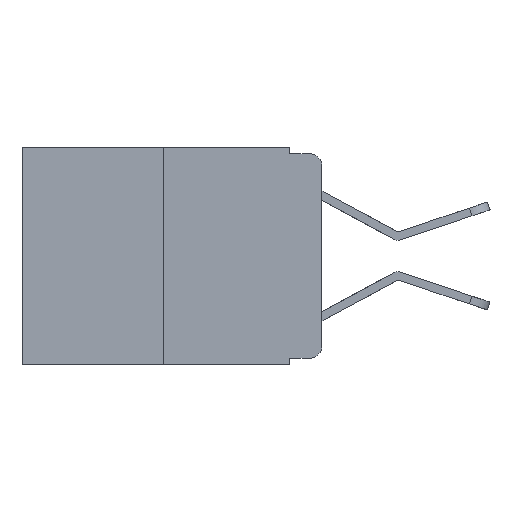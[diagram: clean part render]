
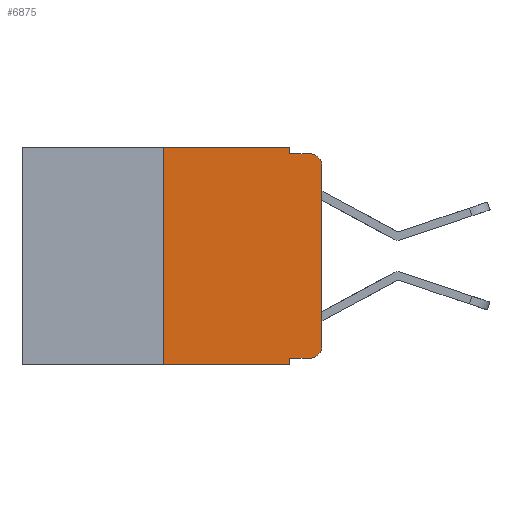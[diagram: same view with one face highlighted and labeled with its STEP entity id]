
A CAD part, left-side view. The second image highlights one B-rep face of the part: STEP entity #6875.
In plain terms, the highlighted planar face has unit normal (-1, 0, 0).
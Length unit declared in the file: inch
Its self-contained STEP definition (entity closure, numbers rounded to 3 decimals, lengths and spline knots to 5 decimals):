
#9 = CARTESIAN_POINT ( 'NONE',  ( 0., 0.25, 0. ) ) ;
#380 = EDGE_CURVE ( 'NONE', #8002, #9967, #12423, .T. ) ;
#555 = VECTOR ( 'NONE', #9686, 39.37008 ) ;
#1324 = DIRECTION ( 'NONE',  ( 0., 0., -1. ) ) ;
#1329 = ORIENTED_EDGE ( 'NONE', *, *, #6156, .F. ) ;
#1380 = EDGE_CURVE ( 'NONE', #8422, #11307, #3279, .T. ) ;
#1679 = LINE ( 'NONE', #6354, #3691 ) ;
#1767 = CARTESIAN_POINT ( 'NONE',  ( 0., 0.051, -0.333 ) ) ;
#1842 = LINE ( 'NONE', #7281, #7123 ) ;
#2035 = VERTEX_POINT ( 'NONE', #9795 ) ;
#2213 = VECTOR ( 'NONE', #10057, 39.37008 ) ;
#2257 = ORIENTED_EDGE ( 'NONE', *, *, #380, .F. ) ;
#2526 = CARTESIAN_POINT ( 'NONE',  ( 0., 0.25, 0. ) ) ;
#2603 = CARTESIAN_POINT ( 'NONE',  ( 0., 0., -0.313 ) ) ;
#2746 = VECTOR ( 'NONE', #3531, 39.37008 ) ;
#2773 = AXIS2_PLACEMENT_3D ( 'NONE', #4020, #6036, #4654 ) ;
#2784 = CIRCLE ( 'NONE', #9295, 0.02 ) ;
#2878 = ORIENTED_EDGE ( 'NONE', *, *, #3241, .T. ) ;
#3169 = VERTEX_POINT ( 'NONE', #2526 ) ;
#3241 = EDGE_CURVE ( 'NONE', #6230, #9994, #2784, .T. ) ;
#3279 = CIRCLE ( 'NONE', #2773, 0.02 ) ;
#3496 = DIRECTION ( 'NONE',  ( 1., 0., 0. ) ) ;
#3519 = CARTESIAN_POINT ( 'NONE',  ( 0., 0.051, -0.343 ) ) ;
#3531 = DIRECTION ( 'NONE',  ( 0., -1., 0. ) ) ;
#3691 = VECTOR ( 'NONE', #10329, 39.37008 ) ;
#3892 = CARTESIAN_POINT ( 'NONE',  ( 0., 0.051, 0. ) ) ;
#4020 = CARTESIAN_POINT ( 'NONE',  ( 0., 0.02, -0.03 ) ) ;
#4257 = DIRECTION ( 'NONE',  ( 0., 0., 1. ) ) ;
#4269 = CARTESIAN_POINT ( 'NONE',  ( 0., 0.051, -0.01 ) ) ;
#4294 = ORIENTED_EDGE ( 'NONE', *, *, #4490, .F. ) ;
#4301 = EDGE_CURVE ( 'NONE', #9994, #8422, #5023, .T. ) ;
#4490 = EDGE_CURVE ( 'NONE', #2035, #3169, #7791, .T. ) ;
#4627 = ORIENTED_EDGE ( 'NONE', *, *, #12728, .T. ) ;
#4654 = DIRECTION ( 'NONE',  ( 0., 0., -1. ) ) ;
#4967 = DIRECTION ( 'NONE',  ( 0., 0., 1. ) ) ;
#5023 = LINE ( 'NONE', #7121, #12544 ) ;
#5165 = VECTOR ( 'NONE', #4967, 39.37008 ) ;
#5235 = LINE ( 'NONE', #4269, #10800 ) ;
#5240 = ORIENTED_EDGE ( 'NONE', *, *, #6415, .T. ) ;
#5496 = DIRECTION ( 'NONE',  ( 0., 0., -1. ) ) ;
#5604 = AXIS2_PLACEMENT_3D ( 'NONE', #7455, #3496, #10445 ) ;
#5696 = ORIENTED_EDGE ( 'NONE', *, *, #4301, .T. ) ;
#6002 = ORIENTED_EDGE ( 'NONE', *, *, #7380, .F. ) ;
#6036 = DIRECTION ( 'NONE',  ( -1., 0., 0. ) ) ;
#6156 = EDGE_CURVE ( 'NONE', #3169, #12342, #1679, .T. ) ;
#6204 = LINE ( 'NONE', #1767, #555 ) ;
#6230 = VERTEX_POINT ( 'NONE', #6479 ) ;
#6354 = CARTESIAN_POINT ( 'NONE',  ( 0., 0.473, 0. ) ) ;
#6415 = EDGE_CURVE ( 'NONE', #8002, #6230, #6204, .T. ) ;
#6479 = CARTESIAN_POINT ( 'NONE',  ( 0., 0.02, -0.333 ) ) ;
#6490 = CARTESIAN_POINT ( 'NONE',  ( 0., 0.02, -0.313 ) ) ;
#6875 = ADVANCED_FACE ( 'NONE', ( #8185 ), #9459, .F. ) ;
#7059 = CARTESIAN_POINT ( 'NONE',  ( 0., 0., -0.03 ) ) ;
#7121 = CARTESIAN_POINT ( 'NONE',  ( 0., 0., 0. ) ) ;
#7123 = VECTOR ( 'NONE', #1324, 39.37008 ) ;
#7281 = CARTESIAN_POINT ( 'NONE',  ( 0., 0.051, 0. ) ) ;
#7380 = EDGE_CURVE ( 'NONE', #10767, #11307, #5235, .T. ) ;
#7455 = CARTESIAN_POINT ( 'NONE',  ( 0., 0.473, 0. ) ) ;
#7791 = LINE ( 'NONE', #9, #5165 ) ;
#8002 = VERTEX_POINT ( 'NONE', #12098 ) ;
#8185 = FACE_OUTER_BOUND ( 'NONE', #11487, .T. ) ;
#8422 = VERTEX_POINT ( 'NONE', #7059 ) ;
#8484 = CARTESIAN_POINT ( 'NONE',  ( 0., 0.473, -0.343 ) ) ;
#9295 = AXIS2_PLACEMENT_3D ( 'NONE', #6490, #12405, #5496 ) ;
#9459 = PLANE ( 'NONE',  #5604 ) ;
#9686 = DIRECTION ( 'NONE',  ( 0., -1., 0. ) ) ;
#9795 = CARTESIAN_POINT ( 'NONE',  ( 0., 0.25, -0.343 ) ) ;
#9967 = VERTEX_POINT ( 'NONE', #3519 ) ;
#9994 = VERTEX_POINT ( 'NONE', #2603 ) ;
#10057 = DIRECTION ( 'NONE',  ( 0., 0., -1. ) ) ;
#10089 = CARTESIAN_POINT ( 'NONE',  ( 0., 0.051, 0. ) ) ;
#10329 = DIRECTION ( 'NONE',  ( 0., -1., 0. ) ) ;
#10445 = DIRECTION ( 'NONE',  ( 0., 0., -1. ) ) ;
#10667 = LINE ( 'NONE', #8484, #2746 ) ;
#10767 = VERTEX_POINT ( 'NONE', #11690 ) ;
#10800 = VECTOR ( 'NONE', #12154, 39.37008 ) ;
#10947 = ORIENTED_EDGE ( 'NONE', *, *, #1380, .T. ) ;
#11247 = ORIENTED_EDGE ( 'NONE', *, *, #11988, .F. ) ;
#11307 = VERTEX_POINT ( 'NONE', #11765 ) ;
#11487 = EDGE_LOOP ( 'NONE', ( #5696, #10947, #6002, #11247, #1329, #4294, #4627, #2257, #5240, #2878 ) ) ;
#11690 = CARTESIAN_POINT ( 'NONE',  ( 0., 0.051, -0.01 ) ) ;
#11765 = CARTESIAN_POINT ( 'NONE',  ( 0., 0.02, -0.01 ) ) ;
#11988 = EDGE_CURVE ( 'NONE', #12342, #10767, #1842, .T. ) ;
#12098 = CARTESIAN_POINT ( 'NONE',  ( 0., 0.051, -0.333 ) ) ;
#12154 = DIRECTION ( 'NONE',  ( 0., -1., 0. ) ) ;
#12342 = VERTEX_POINT ( 'NONE', #3892 ) ;
#12405 = DIRECTION ( 'NONE',  ( -1., 0., 0. ) ) ;
#12423 = LINE ( 'NONE', #10089, #2213 ) ;
#12544 = VECTOR ( 'NONE', #4257, 39.37008 ) ;
#12728 = EDGE_CURVE ( 'NONE', #2035, #9967, #10667, .T. ) ;
